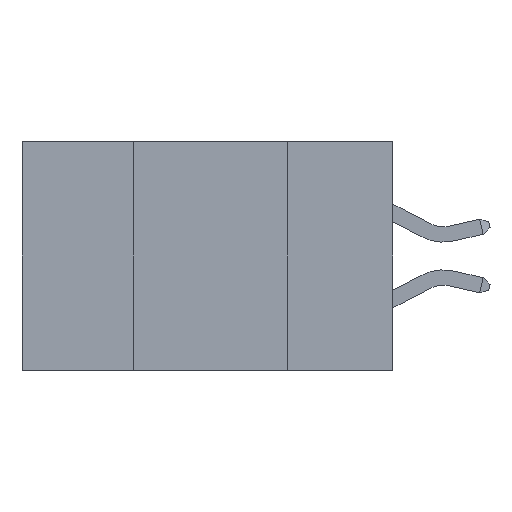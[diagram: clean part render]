
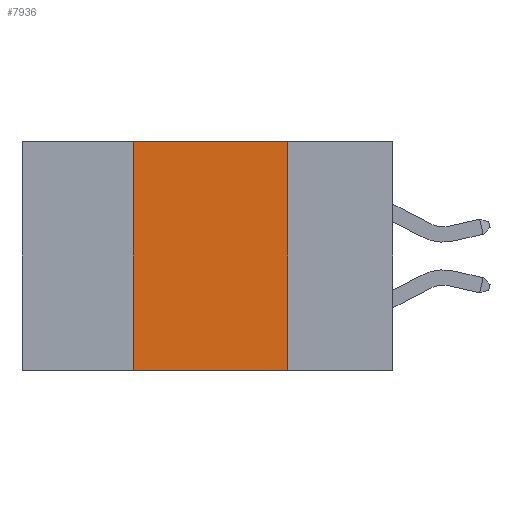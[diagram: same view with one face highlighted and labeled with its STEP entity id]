
A CAD part, left-side view. The second image highlights one B-rep face of the part: STEP entity #7936.
In plain terms, the highlighted planar face has unit normal (-1, 0, 0).
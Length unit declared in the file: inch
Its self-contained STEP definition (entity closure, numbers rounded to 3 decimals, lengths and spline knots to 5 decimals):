
#2352 = DIRECTION ( 'NONE',  ( 0., 0., -1. ) ) ;
#4223 = CARTESIAN_POINT ( 'NONE',  ( 0., 0.17, -0.37 ) ) ;
#6023 = ORIENTED_EDGE ( 'NONE', *, *, #21378, .F. ) ;
#7694 = AXIS2_PLACEMENT_3D ( 'NONE', #26766, #10725, #13635 ) ;
#7936 = ADVANCED_FACE ( 'NONE', ( #34291 ), #29664, .F. ) ;
#8446 = VECTOR ( 'NONE', #19554, 39.37008 ) ;
#9294 = LINE ( 'NONE', #27967, #8446 ) ;
#9755 = CARTESIAN_POINT ( 'NONE',  ( 0., 0.42, 0. ) ) ;
#9979 = VECTOR ( 'NONE', #2352, 39.37008 ) ;
#10691 = VECTOR ( 'NONE', #11445, 39.37008 ) ;
#10725 = DIRECTION ( 'NONE',  ( 1., 0., 0. ) ) ;
#11445 = DIRECTION ( 'NONE',  ( 0., -1., 0. ) ) ;
#12889 = VERTEX_POINT ( 'NONE', #9755 ) ;
#13018 = EDGE_LOOP ( 'NONE', ( #6023, #16827, #15180, #16287 ) ) ;
#13635 = DIRECTION ( 'NONE',  ( 0., 0., -1. ) ) ;
#14618 = DIRECTION ( 'NONE',  ( 0., -1., 0. ) ) ;
#15180 = ORIENTED_EDGE ( 'NONE', *, *, #25874, .F. ) ;
#16287 = ORIENTED_EDGE ( 'NONE', *, *, #16773, .T. ) ;
#16773 = EDGE_CURVE ( 'NONE', #17244, #28562, #29510, .T. ) ;
#16827 = ORIENTED_EDGE ( 'NONE', *, *, #19192, .F. ) ;
#17244 = VERTEX_POINT ( 'NONE', #27447 ) ;
#18383 = CARTESIAN_POINT ( 'NONE',  ( 0., 0.17, 0. ) ) ;
#18931 = VECTOR ( 'NONE', #14618, 39.37008 ) ;
#19192 = EDGE_CURVE ( 'NONE', #12889, #19524, #26062, .T. ) ;
#19524 = VERTEX_POINT ( 'NONE', #28594 ) ;
#19554 = DIRECTION ( 'NONE',  ( 0., 0., 1. ) ) ;
#21245 = CARTESIAN_POINT ( 'NONE',  ( 0., 0.6, 0. ) ) ;
#21378 = EDGE_CURVE ( 'NONE', #19524, #28562, #24195, .T. ) ;
#24195 = LINE ( 'NONE', #18383, #9979 ) ;
#25874 = EDGE_CURVE ( 'NONE', #17244, #12889, #9294, .T. ) ;
#26062 = LINE ( 'NONE', #21245, #18931 ) ;
#26766 = CARTESIAN_POINT ( 'NONE',  ( 0., 0.6, 0. ) ) ;
#27447 = CARTESIAN_POINT ( 'NONE',  ( 0., 0.42, -0.37 ) ) ;
#27721 = CARTESIAN_POINT ( 'NONE',  ( 0., 0.6, -0.37 ) ) ;
#27967 = CARTESIAN_POINT ( 'NONE',  ( 0., 0.42, 0. ) ) ;
#28562 = VERTEX_POINT ( 'NONE', #4223 ) ;
#28594 = CARTESIAN_POINT ( 'NONE',  ( 0., 0.17, 0. ) ) ;
#29510 = LINE ( 'NONE', #27721, #10691 ) ;
#29664 = PLANE ( 'NONE',  #7694 ) ;
#34291 = FACE_OUTER_BOUND ( 'NONE', #13018, .T. ) ;
